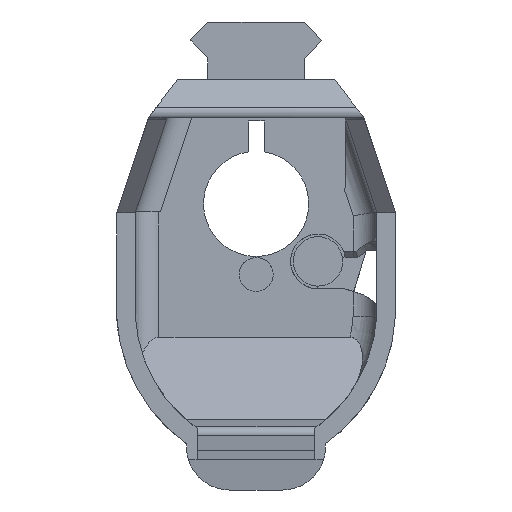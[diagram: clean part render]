
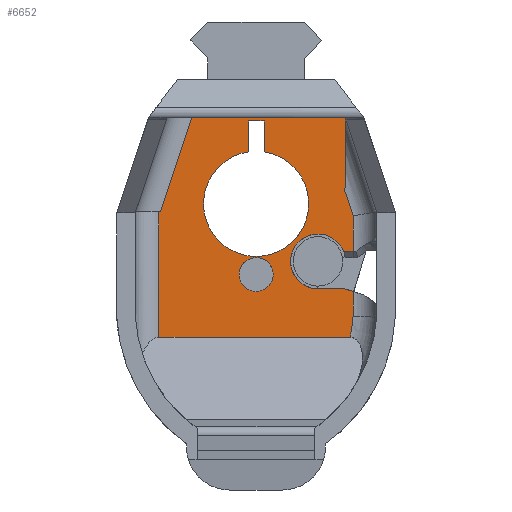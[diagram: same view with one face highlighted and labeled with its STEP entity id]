
A CAD part, front view. The second image highlights one B-rep face of the part: STEP entity #6652.
In plain terms, the highlighted planar face has unit normal (0, -1, 0).
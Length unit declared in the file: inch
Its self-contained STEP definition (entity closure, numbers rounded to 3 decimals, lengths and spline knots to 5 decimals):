
#52=FACE_BOUND('',#842,.T.);
#53=FACE_BOUND('',#843,.T.);
#66=CIRCLE('',#6919,0.33465);
#68=CIRCLE('',#6924,0.17421);
#72=CIRCLE('',#6932,0.10827);
#73=CIRCLE('',#6933,0.10827);
#99=CIRCLE('',#7099,0.78536);
#489=FACE_OUTER_BOUND('',#841,.T.);
#841=EDGE_LOOP('',(#5643,#5644,#5645,#5646,#5647,#5648,#5649,#5650,#5651,
#5652,#5653,#5654,#5655,#5656,#5657,#5658));
#842=EDGE_LOOP('',(#5659,#5660));
#843=EDGE_LOOP('',(#5661,#5662,#5663,#5664));
#1350=LINE('',#9887,#2178);
#1432=LINE('',#10189,#2260);
#1448=LINE('',#10221,#2276);
#1454=LINE('',#10239,#2282);
#1459=LINE('',#10249,#2287);
#1575=LINE('',#10570,#2403);
#1576=LINE('',#10574,#2404);
#1630=LINE('',#10692,#2458);
#1638=LINE('',#10707,#2466);
#1641=LINE('',#10745,#2469);
#1642=LINE('',#10748,#2470);
#1643=LINE('',#10751,#2471);
#1644=LINE('',#10753,#2472);
#1645=LINE('',#10757,#2473);
#1646=LINE('',#10758,#2474);
#1647=LINE('',#10760,#2475);
#1648=LINE('',#10761,#2476);
#2178=VECTOR('',#7975,0.3937);
#2260=VECTOR('',#8183,0.3937);
#2276=VECTOR('',#8209,0.3937);
#2282=VECTOR('',#8225,0.3937);
#2287=VECTOR('',#8232,0.3937);
#2403=VECTOR('',#8510,0.3937);
#2404=VECTOR('',#8515,0.3937);
#2458=VECTOR('',#8617,0.3937);
#2466=VECTOR('',#8631,0.3937);
#2469=VECTOR('',#8644,0.3937);
#2470=VECTOR('',#8647,0.3937);
#2471=VECTOR('',#8652,0.3937);
#2472=VECTOR('',#8653,0.3937);
#2473=VECTOR('',#8656,0.3937);
#2474=VECTOR('',#8657,0.3937);
#2475=VECTOR('',#8658,0.3937);
#2476=VECTOR('',#8659,0.3937);
#2849=VERTEX_POINT('',#9880);
#2852=VERTEX_POINT('',#9885);
#2878=VERTEX_POINT('',#9951);
#2879=VERTEX_POINT('',#9953);
#2895=VERTEX_POINT('',#10023);
#2900=VERTEX_POINT('',#10040);
#2901=VERTEX_POINT('',#10041);
#2947=VERTEX_POINT('',#10186);
#2948=VERTEX_POINT('',#10188);
#2959=VERTEX_POINT('',#10219);
#2965=VERTEX_POINT('',#10237);
#2966=VERTEX_POINT('',#10238);
#2970=VERTEX_POINT('',#10248);
#3064=VERTEX_POINT('',#10568);
#3065=VERTEX_POINT('',#10572);
#3105=VERTEX_POINT('',#10691);
#3113=VERTEX_POINT('',#10743);
#3114=VERTEX_POINT('',#10747);
#3115=VERTEX_POINT('',#10752);
#3116=VERTEX_POINT('',#10754);
#3117=VERTEX_POINT('',#10756);
#3118=VERTEX_POINT('',#10759);
#3622=EDGE_CURVE('',#2852,#2849,#1350,.T.);
#3654=EDGE_CURVE('',#2879,#2878,#66,.T.);
#3673=EDGE_CURVE('',#2895,#2849,#68,.T.);
#3679=EDGE_CURVE('',#2900,#2901,#72,.T.);
#3680=EDGE_CURVE('',#2901,#2900,#73,.T.);
#3742=EDGE_CURVE('',#2947,#2948,#1432,.T.);
#3759=EDGE_CURVE('',#2959,#2895,#1448,.T.);
#3767=EDGE_CURVE('',#2965,#2966,#1454,.T.);
#3772=EDGE_CURVE('',#2970,#2966,#1459,.T.);
#3926=EDGE_CURVE('',#2965,#3064,#1575,.T.);
#3928=EDGE_CURVE('',#3064,#3065,#1576,.T.);
#3989=EDGE_CURVE('',#3105,#2879,#1630,.T.);
#3998=EDGE_CURVE('',#2948,#3065,#1638,.T.);
#4006=EDGE_CURVE('',#3113,#2947,#1641,.T.);
#4007=EDGE_CURVE('',#2970,#3114,#1642,.T.);
#4009=EDGE_CURVE('',#3114,#2852,#1643,.T.);
#4010=EDGE_CURVE('',#3113,#3115,#1644,.T.);
#4011=EDGE_CURVE('',#3116,#3115,#99,.T.);
#4012=EDGE_CURVE('',#3117,#3116,#1645,.T.);
#4013=EDGE_CURVE('',#2959,#3117,#1646,.T.);
#4014=EDGE_CURVE('',#2878,#3118,#1647,.T.);
#4015=EDGE_CURVE('',#3118,#3105,#1648,.T.);
#5643=ORIENTED_EDGE('',*,*,#3622,.F.);
#5644=ORIENTED_EDGE('',*,*,#4009,.F.);
#5645=ORIENTED_EDGE('',*,*,#4007,.F.);
#5646=ORIENTED_EDGE('',*,*,#3772,.T.);
#5647=ORIENTED_EDGE('',*,*,#3767,.F.);
#5648=ORIENTED_EDGE('',*,*,#3926,.T.);
#5649=ORIENTED_EDGE('',*,*,#3928,.T.);
#5650=ORIENTED_EDGE('',*,*,#3998,.F.);
#5651=ORIENTED_EDGE('',*,*,#3742,.F.);
#5652=ORIENTED_EDGE('',*,*,#4006,.F.);
#5653=ORIENTED_EDGE('',*,*,#4010,.T.);
#5654=ORIENTED_EDGE('',*,*,#4011,.F.);
#5655=ORIENTED_EDGE('',*,*,#4012,.F.);
#5656=ORIENTED_EDGE('',*,*,#4013,.F.);
#5657=ORIENTED_EDGE('',*,*,#3759,.T.);
#5658=ORIENTED_EDGE('',*,*,#3673,.T.);
#5659=ORIENTED_EDGE('',*,*,#3679,.T.);
#5660=ORIENTED_EDGE('',*,*,#3680,.T.);
#5661=ORIENTED_EDGE('',*,*,#3989,.T.);
#5662=ORIENTED_EDGE('',*,*,#3654,.T.);
#5663=ORIENTED_EDGE('',*,*,#4014,.T.);
#5664=ORIENTED_EDGE('',*,*,#4015,.T.);
#6322=PLANE('',#7098);
#6652=ADVANCED_FACE('',(#489,#52,#53),#6322,.T.);
#6919=AXIS2_PLACEMENT_3D('',#9954,#8024,#8025);
#6924=AXIS2_PLACEMENT_3D('',#10027,#8049,#8050);
#6932=AXIS2_PLACEMENT_3D('',#10042,#8067,#8068);
#6933=AXIS2_PLACEMENT_3D('',#10043,#8069,#8070);
#7098=AXIS2_PLACEMENT_3D('',#10750,#8650,#8651);
#7099=AXIS2_PLACEMENT_3D('',#10755,#8654,#8655);
#7975=DIRECTION('',(-1.,0.,0.));
#8024=DIRECTION('center_axis',(0.,1.,0.));
#8025=DIRECTION('ref_axis',(-1.,0.,0.));
#8049=DIRECTION('center_axis',(0.,1.,0.));
#8050=DIRECTION('ref_axis',(1.,0.,0.));
#8067=DIRECTION('center_axis',(0.,1.,0.));
#8068=DIRECTION('ref_axis',(1.,0.,0.));
#8069=DIRECTION('center_axis',(0.,1.,0.));
#8070=DIRECTION('ref_axis',(1.,0.,0.));
#8183=DIRECTION('',(1.,0.,0.));
#8209=DIRECTION('',(-1.,0.,0.));
#8225=DIRECTION('',(1.,0.,-0.002));
#8232=DIRECTION('',(0.002,0.,1.));
#8510=DIRECTION('',(0.,0.,-1.));
#8515=DIRECTION('',(-1.,0.,0.));
#8617=DIRECTION('',(0.,0.,-1.));
#8631=DIRECTION('',(0.316,0.,0.949));
#8644=DIRECTION('',(0.,0.,1.));
#8647=DIRECTION('',(0.316,0.,-0.949));
#8650=DIRECTION('center_axis',(0.,-1.,0.));
#8651=DIRECTION('ref_axis',(0.,0.,-1.));
#8652=DIRECTION('',(0.,0.,-1.));
#8653=DIRECTION('',(1.,0.,0.));
#8654=DIRECTION('center_axis',(0.,1.,0.));
#8655=DIRECTION('ref_axis',(0.992,0.,-0.128));
#8656=DIRECTION('',(0.,0.,-1.));
#8657=DIRECTION('',(0.954,0.,-0.301));
#8658=DIRECTION('',(0.,0.,1.));
#8659=DIRECTION('',(1.,0.,0.));
#9880=CARTESIAN_POINT('',(0.55575,2.56,0.14773));
#9885=CARTESIAN_POINT('',(0.61679,2.56,0.14773));
#9887=CARTESIAN_POINT('',(0.03313,2.56,0.14773));
#9951=CARTESIAN_POINT('',(-0.0477,2.56,0.78123));
#9953=CARTESIAN_POINT('',(0.05072,2.56,0.78078));
#9954=CARTESIAN_POINT('Origin',(0.,2.56,0.45));
#10023=CARTESIAN_POINT('',(0.41433,2.56,-0.08921));
#10027=CARTESIAN_POINT('Origin',(0.3937,2.56,0.08378));
#10040=CARTESIAN_POINT('',(-0.05174,2.56,0.0951));
#10041=CARTESIAN_POINT('',(-0.10827,2.56,0.));
#10042=CARTESIAN_POINT('Origin',(0.,2.56,0.));
#10043=CARTESIAN_POINT('Origin',(0.,2.56,0.));
#10186=CARTESIAN_POINT('',(-0.61864,2.56,0.39831));
#10188=CARTESIAN_POINT('',(-0.60868,2.56,0.39831));
#10189=CARTESIAN_POINT('',(-0.79245,2.56,0.39831));
#10219=CARTESIAN_POINT('',(0.55783,2.56,-0.08921));
#10221=CARTESIAN_POINT('',(0.10264,2.56,-0.08921));
#10237=CARTESIAN_POINT('',(0.5,2.56,1.0001));
#10238=CARTESIAN_POINT('',(0.56627,2.56,0.99997));
#10239=CARTESIAN_POINT('',(0.5,2.56,1.0001));
#10248=CARTESIAN_POINT('',(0.56534,2.56,0.52831));
#10249=CARTESIAN_POINT('',(0.56627,2.56,0.99987));
#10568=CARTESIAN_POINT('',(0.5,2.56,0.99982));
#10570=CARTESIAN_POINT('',(0.5,2.56,0.64988));
#10572=CARTESIAN_POINT('',(-0.40817,2.56,0.99982));
#10574=CARTESIAN_POINT('',(-0.5,2.56,0.99982));
#10691=CARTESIAN_POINT('',(0.05072,2.56,0.97719));
#10692=CARTESIAN_POINT('',(0.05072,2.56,0.54014));
#10707=CARTESIAN_POINT('',(-0.6259,2.56,0.34662));
#10743=CARTESIAN_POINT('',(-0.61864,2.56,-0.4));
#10745=CARTESIAN_POINT('',(-0.61864,2.56,0.34912));
#10747=CARTESIAN_POINT('',(0.61679,2.56,0.37396));
#10748=CARTESIAN_POINT('',(0.47564,2.56,0.79741));
#10750=CARTESIAN_POINT('Origin',(-0.5,2.56,0.29994));
#10751=CARTESIAN_POINT('',(0.61679,2.56,0.01448));
#10752=CARTESIAN_POINT('',(0.59654,2.56,-0.4));
#10753=CARTESIAN_POINT('',(0.37309,2.56,-0.4));
#10754=CARTESIAN_POINT('',(0.61679,2.56,-0.26638));
#10755=CARTESIAN_POINT('Origin',(-0.16695,2.56,-0.21593));
#10756=CARTESIAN_POINT('',(0.61679,2.56,-0.1078));
#10757=CARTESIAN_POINT('',(0.61679,2.56,0.01448));
#10758=CARTESIAN_POINT('',(0.05278,2.56,0.07004));
#10759=CARTESIAN_POINT('',(-0.0477,2.56,0.97719));
#10760=CARTESIAN_POINT('',(-0.0477,2.56,0.54014));
#10761=CARTESIAN_POINT('',(-0.22464,2.56,0.97719));
